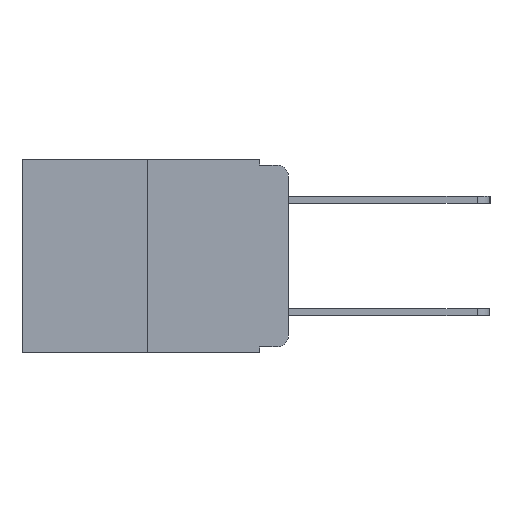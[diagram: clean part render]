
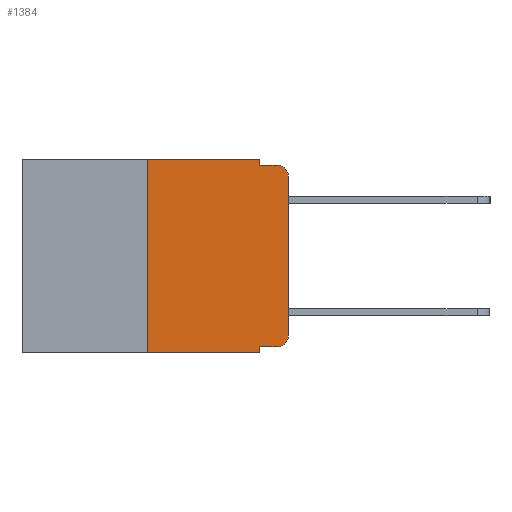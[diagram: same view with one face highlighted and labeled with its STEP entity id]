
A CAD part, left-side view. The second image highlights one B-rep face of the part: STEP entity #1384.
In plain terms, the highlighted planar face has unit normal (-1, 0, 0).
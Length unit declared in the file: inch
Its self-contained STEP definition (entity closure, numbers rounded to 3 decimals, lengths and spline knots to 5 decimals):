
#280 = VECTOR ( 'NONE', #4006, 39.37008 ) ;
#360 = CARTESIAN_POINT ( 'NONE',  ( 0., 0., -0.313 ) ) ;
#412 = DIRECTION ( 'NONE',  ( 0., 0., -1. ) ) ;
#448 = DIRECTION ( 'NONE',  ( -1., 0., 0. ) ) ;
#558 = CARTESIAN_POINT ( 'NONE',  ( 0., 0.02, -0.313 ) ) ;
#561 = VECTOR ( 'NONE', #6796, 39.37008 ) ;
#697 = LINE ( 'NONE', #2999, #280 ) ;
#726 = DIRECTION ( 'NONE',  ( 0., 0., -1. ) ) ;
#1109 = CARTESIAN_POINT ( 'NONE',  ( 0., 0.02, -0.333 ) ) ;
#1384 = ADVANCED_FACE ( 'NONE', ( #8898 ), #9933, .F. ) ;
#1651 = VECTOR ( 'NONE', #10699, 39.37008 ) ;
#2070 = VERTEX_POINT ( 'NONE', #360 ) ;
#2116 = VECTOR ( 'NONE', #3077, 39.37008 ) ;
#2249 = ORIENTED_EDGE ( 'NONE', *, *, #7298, .T. ) ;
#2424 = CARTESIAN_POINT ( 'NONE',  ( 0., 0.051, -0.01 ) ) ;
#2814 = LINE ( 'NONE', #12141, #2116 ) ;
#2852 = VERTEX_POINT ( 'NONE', #10581 ) ;
#2894 = ORIENTED_EDGE ( 'NONE', *, *, #6290, .F. ) ;
#2999 = CARTESIAN_POINT ( 'NONE',  ( 0., 0.473, 0. ) ) ;
#3077 = DIRECTION ( 'NONE',  ( 0., 0., 1. ) ) ;
#3208 = DIRECTION ( 'NONE',  ( 0., 0., -1. ) ) ;
#3229 = ORIENTED_EDGE ( 'NONE', *, *, #9041, .F. ) ;
#3347 = CARTESIAN_POINT ( 'NONE',  ( 0., 0.473, -0.343 ) ) ;
#3426 = AXIS2_PLACEMENT_3D ( 'NONE', #7672, #11592, #10519 ) ;
#3542 = VERTEX_POINT ( 'NONE', #4831 ) ;
#3573 = LINE ( 'NONE', #2424, #561 ) ;
#3806 = EDGE_CURVE ( 'NONE', #9266, #10855, #3573, .T. ) ;
#4006 = DIRECTION ( 'NONE',  ( 0., -1., 0. ) ) ;
#4096 = DIRECTION ( 'NONE',  ( 0., 0., -1. ) ) ;
#4138 = LINE ( 'NONE', #10389, #8814 ) ;
#4279 = LINE ( 'NONE', #8155, #8942 ) ;
#4698 = EDGE_CURVE ( 'NONE', #9675, #2070, #12440, .T. ) ;
#4831 = CARTESIAN_POINT ( 'NONE',  ( 0., 0.25, 0. ) ) ;
#4970 = VERTEX_POINT ( 'NONE', #6584 ) ;
#5166 = ORIENTED_EDGE ( 'NONE', *, *, #12458, .F. ) ;
#5218 = CARTESIAN_POINT ( 'NONE',  ( 0., 0.02, -0.01 ) ) ;
#5315 = VERTEX_POINT ( 'NONE', #7019 ) ;
#5613 = LINE ( 'NONE', #12245, #7791 ) ;
#5770 = CARTESIAN_POINT ( 'NONE',  ( 0., 0.051, -0.333 ) ) ;
#5908 = CARTESIAN_POINT ( 'NONE',  ( 0., 0.25, -0.343 ) ) ;
#5932 = EDGE_CURVE ( 'NONE', #11527, #9675, #4138, .T. ) ;
#6190 = ORIENTED_EDGE ( 'NONE', *, *, #11684, .T. ) ;
#6290 = EDGE_CURVE ( 'NONE', #3542, #4970, #697, .T. ) ;
#6306 = EDGE_CURVE ( 'NONE', #2852, #10855, #8375, .T. ) ;
#6584 = CARTESIAN_POINT ( 'NONE',  ( 0., 0.051, 0. ) ) ;
#6796 = DIRECTION ( 'NONE',  ( 0., -1., 0. ) ) ;
#6835 = DIRECTION ( 'NONE',  ( -1., 0., 0. ) ) ;
#6850 = VECTOR ( 'NONE', #4096, 39.37008 ) ;
#6906 = ORIENTED_EDGE ( 'NONE', *, *, #6306, .T. ) ;
#7019 = CARTESIAN_POINT ( 'NONE',  ( 0., 0.051, -0.343 ) ) ;
#7168 = EDGE_CURVE ( 'NONE', #11527, #5315, #5613, .T. ) ;
#7298 = EDGE_CURVE ( 'NONE', #12434, #5315, #11353, .T. ) ;
#7498 = CARTESIAN_POINT ( 'NONE',  ( 0., 0.051, -0.01 ) ) ;
#7672 = CARTESIAN_POINT ( 'NONE',  ( 0., 0.473, 0. ) ) ;
#7791 = VECTOR ( 'NONE', #3208, 39.37008 ) ;
#7824 = CARTESIAN_POINT ( 'NONE',  ( 0., 0.051, 0. ) ) ;
#8155 = CARTESIAN_POINT ( 'NONE',  ( 0., 0.25, 0. ) ) ;
#8375 = CIRCLE ( 'NONE', #10360, 0.02 ) ;
#8814 = VECTOR ( 'NONE', #10024, 39.37008 ) ;
#8898 = FACE_OUTER_BOUND ( 'NONE', #11818, .T. ) ;
#8942 = VECTOR ( 'NONE', #9082, 39.37008 ) ;
#9041 = EDGE_CURVE ( 'NONE', #12434, #3542, #4279, .T. ) ;
#9082 = DIRECTION ( 'NONE',  ( 0., 0., 1. ) ) ;
#9266 = VERTEX_POINT ( 'NONE', #7498 ) ;
#9305 = LINE ( 'NONE', #7824, #6850 ) ;
#9556 = ORIENTED_EDGE ( 'NONE', *, *, #7168, .F. ) ;
#9675 = VERTEX_POINT ( 'NONE', #1109 ) ;
#9933 = PLANE ( 'NONE',  #3426 ) ;
#10024 = DIRECTION ( 'NONE',  ( 0., -1., 0. ) ) ;
#10360 = AXIS2_PLACEMENT_3D ( 'NONE', #12119, #6835, #726 ) ;
#10389 = CARTESIAN_POINT ( 'NONE',  ( 0., 0.051, -0.333 ) ) ;
#10506 = ORIENTED_EDGE ( 'NONE', *, *, #4698, .T. ) ;
#10519 = DIRECTION ( 'NONE',  ( 0., 0., -1. ) ) ;
#10581 = CARTESIAN_POINT ( 'NONE',  ( 0., 0., -0.03 ) ) ;
#10699 = DIRECTION ( 'NONE',  ( 0., -1., 0. ) ) ;
#10840 = ORIENTED_EDGE ( 'NONE', *, *, #3806, .F. ) ;
#10855 = VERTEX_POINT ( 'NONE', #5218 ) ;
#11136 = ORIENTED_EDGE ( 'NONE', *, *, #5932, .T. ) ;
#11333 = AXIS2_PLACEMENT_3D ( 'NONE', #558, #448, #412 ) ;
#11353 = LINE ( 'NONE', #3347, #1651 ) ;
#11527 = VERTEX_POINT ( 'NONE', #5770 ) ;
#11592 = DIRECTION ( 'NONE',  ( 1., 0., 0. ) ) ;
#11684 = EDGE_CURVE ( 'NONE', #2070, #2852, #2814, .T. ) ;
#11818 = EDGE_LOOP ( 'NONE', ( #6190, #6906, #10840, #5166, #2894, #3229, #2249, #9556, #11136, #10506 ) ) ;
#12119 = CARTESIAN_POINT ( 'NONE',  ( 0., 0.02, -0.03 ) ) ;
#12141 = CARTESIAN_POINT ( 'NONE',  ( 0., 0., 0. ) ) ;
#12245 = CARTESIAN_POINT ( 'NONE',  ( 0., 0.051, 0. ) ) ;
#12434 = VERTEX_POINT ( 'NONE', #5908 ) ;
#12440 = CIRCLE ( 'NONE', #11333, 0.02 ) ;
#12458 = EDGE_CURVE ( 'NONE', #4970, #9266, #9305, .T. ) ;
